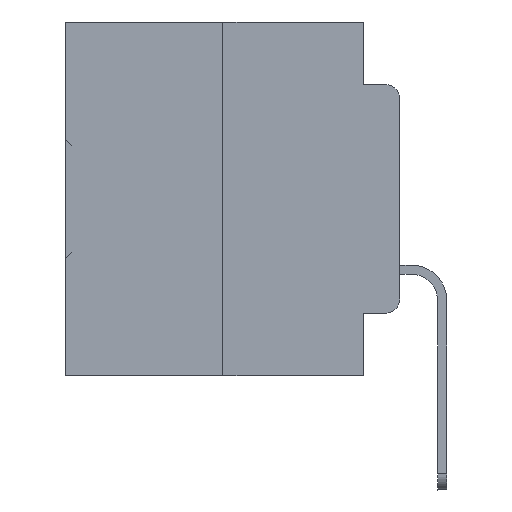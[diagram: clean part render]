
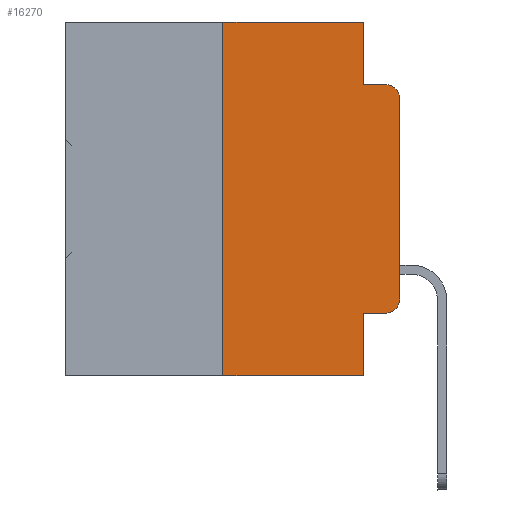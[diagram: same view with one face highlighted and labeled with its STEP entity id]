
A CAD part, left-side view. The second image highlights one B-rep face of the part: STEP entity #16270.
In plain terms, the highlighted planar face has unit normal (-1, 0, 0).
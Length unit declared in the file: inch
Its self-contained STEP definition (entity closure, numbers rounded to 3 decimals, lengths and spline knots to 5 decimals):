
#1047 = DIRECTION ( 'NONE',  ( 0., -1., 0. ) ) ;
#1428 = VERTEX_POINT ( 'NONE', #19701 ) ;
#2067 = AXIS2_PLACEMENT_3D ( 'NONE', #17730, #5120, #20406 ) ;
#2646 = LINE ( 'NONE', #24477, #24398 ) ;
#2714 = VECTOR ( 'NONE', #7329, 39.37008 ) ;
#2801 = CARTESIAN_POINT ( 'NONE',  ( 0., 0.051, -0.4115 ) ) ;
#3658 = CARTESIAN_POINT ( 'NONE',  ( 0., 0.051, 0. ) ) ;
#3923 = EDGE_CURVE ( 'NONE', #4097, #30603, #10318, .T. ) ;
#4097 = VERTEX_POINT ( 'NONE', #33542 ) ;
#4392 = ORIENTED_EDGE ( 'NONE', *, *, #19052, .T. ) ;
#4418 = CARTESIAN_POINT ( 'NONE',  ( 0., 0.473, 0. ) ) ;
#5120 = DIRECTION ( 'NONE',  ( -1., 0., 0. ) ) ;
#6440 = AXIS2_PLACEMENT_3D ( 'NONE', #33816, #31138, #26849 ) ;
#6537 = CARTESIAN_POINT ( 'NONE',  ( 0., 0.051, 0. ) ) ;
#7329 = DIRECTION ( 'NONE',  ( 0., 0., -1. ) ) ;
#7428 = EDGE_CURVE ( 'NONE', #25751, #30376, #25580, .T. ) ;
#8177 = DIRECTION ( 'NONE',  ( 0., 0., -1. ) ) ;
#8266 = CARTESIAN_POINT ( 'NONE',  ( 0., 0., 0. ) ) ;
#8696 = CARTESIAN_POINT ( 'NONE',  ( 0., 0.02, -0.3915 ) ) ;
#10022 = LINE ( 'NONE', #2801, #25629 ) ;
#10318 = LINE ( 'NONE', #4418, #25053 ) ;
#10755 = VECTOR ( 'NONE', #1047, 39.37008 ) ;
#11928 = DIRECTION ( 'NONE',  ( 0., 0., -1. ) ) ;
#12005 = PLANE ( 'NONE',  #6440 ) ;
#12244 = ORIENTED_EDGE ( 'NONE', *, *, #13555, .F. ) ;
#12829 = CIRCLE ( 'NONE', #16283, 0.02 ) ;
#13066 = LINE ( 'NONE', #26654, #2714 ) ;
#13218 = DIRECTION ( 'NONE',  ( 0., 0., 1. ) ) ;
#13371 = DIRECTION ( 'NONE',  ( 0., -1., 0. ) ) ;
#13555 = EDGE_CURVE ( 'NONE', #28451, #1428, #25912, .T. ) ;
#14150 = VERTEX_POINT ( 'NONE', #16201 ) ;
#14521 = CARTESIAN_POINT ( 'NONE',  ( 0., 0.02, -0.4115 ) ) ;
#14811 = ORIENTED_EDGE ( 'NONE', *, *, #21193, .F. ) ;
#16160 = DIRECTION ( 'NONE',  ( 0., 0., 1. ) ) ;
#16201 = CARTESIAN_POINT ( 'NONE',  ( 0., 0., -0.1085 ) ) ;
#16270 = ADVANCED_FACE ( 'NONE', ( #22268 ), #12005, .F. ) ;
#16283 = AXIS2_PLACEMENT_3D ( 'NONE', #8696, #22149, #8177 ) ;
#16570 = VERTEX_POINT ( 'NONE', #20389 ) ;
#16969 = EDGE_CURVE ( 'NONE', #30603, #28451, #33043, .T. ) ;
#17385 = ORIENTED_EDGE ( 'NONE', *, *, #7428, .T. ) ;
#17545 = CARTESIAN_POINT ( 'NONE',  ( 0., 0.473, -0.5 ) ) ;
#17730 = CARTESIAN_POINT ( 'NONE',  ( 0., 0.02, -0.1085 ) ) ;
#18510 = LINE ( 'NONE', #8266, #28901 ) ;
#19052 = EDGE_CURVE ( 'NONE', #24013, #14150, #18510, .T. ) ;
#19184 = VERTEX_POINT ( 'NONE', #14521 ) ;
#19273 = ORIENTED_EDGE ( 'NONE', *, *, #34750, .F. ) ;
#19701 = CARTESIAN_POINT ( 'NONE',  ( 0., 0.02, -0.0885 ) ) ;
#20038 = CARTESIAN_POINT ( 'NONE',  ( 0., 0.051, -0.0885 ) ) ;
#20389 = CARTESIAN_POINT ( 'NONE',  ( 0., 0.051, -0.4115 ) ) ;
#20406 = DIRECTION ( 'NONE',  ( 0., 0., -1. ) ) ;
#21034 = ORIENTED_EDGE ( 'NONE', *, *, #16969, .F. ) ;
#21193 = EDGE_CURVE ( 'NONE', #16570, #30376, #13066, .T. ) ;
#21410 = CARTESIAN_POINT ( 'NONE',  ( 0., 0.051, -0.5 ) ) ;
#22149 = DIRECTION ( 'NONE',  ( -1., 0., 0. ) ) ;
#22268 = FACE_OUTER_BOUND ( 'NONE', #26660, .T. ) ;
#22275 = ORIENTED_EDGE ( 'NONE', *, *, #27135, .T. ) ;
#23628 = VECTOR ( 'NONE', #11928, 39.37008 ) ;
#23956 = EDGE_CURVE ( 'NONE', #16570, #19184, #10022, .T. ) ;
#24013 = VERTEX_POINT ( 'NONE', #27140 ) ;
#24398 = VECTOR ( 'NONE', #13218, 39.37008 ) ;
#24477 = CARTESIAN_POINT ( 'NONE',  ( 0., 0.25, 0. ) ) ;
#25053 = VECTOR ( 'NONE', #29101, 39.37008 ) ;
#25580 = LINE ( 'NONE', #17545, #10755 ) ;
#25629 = VECTOR ( 'NONE', #13371, 39.37008 ) ;
#25751 = VERTEX_POINT ( 'NONE', #32159 ) ;
#25912 = LINE ( 'NONE', #31627, #34396 ) ;
#26654 = CARTESIAN_POINT ( 'NONE',  ( 0., 0.051, 0. ) ) ;
#26660 = EDGE_LOOP ( 'NONE', ( #4392, #27583, #12244, #21034, #34229, #19273, #17385, #14811, #32820, #22275 ) ) ;
#26849 = DIRECTION ( 'NONE',  ( 0., 0., -1. ) ) ;
#27135 = EDGE_CURVE ( 'NONE', #19184, #24013, #12829, .T. ) ;
#27140 = CARTESIAN_POINT ( 'NONE',  ( 0., 0., -0.3915 ) ) ;
#27583 = ORIENTED_EDGE ( 'NONE', *, *, #30368, .T. ) ;
#28451 = VERTEX_POINT ( 'NONE', #20038 ) ;
#28901 = VECTOR ( 'NONE', #16160, 39.37008 ) ;
#29101 = DIRECTION ( 'NONE',  ( 0., -1., 0. ) ) ;
#30368 = EDGE_CURVE ( 'NONE', #14150, #1428, #32911, .T. ) ;
#30376 = VERTEX_POINT ( 'NONE', #21410 ) ;
#30603 = VERTEX_POINT ( 'NONE', #3658 ) ;
#31088 = DIRECTION ( 'NONE',  ( 0., -1., 0. ) ) ;
#31138 = DIRECTION ( 'NONE',  ( 1., 0., 0. ) ) ;
#31627 = CARTESIAN_POINT ( 'NONE',  ( 0., 0.051, -0.0885 ) ) ;
#32159 = CARTESIAN_POINT ( 'NONE',  ( 0., 0.25, -0.5 ) ) ;
#32820 = ORIENTED_EDGE ( 'NONE', *, *, #23956, .T. ) ;
#32911 = CIRCLE ( 'NONE', #2067, 0.02 ) ;
#33043 = LINE ( 'NONE', #6537, #23628 ) ;
#33542 = CARTESIAN_POINT ( 'NONE',  ( 0., 0.25, 0. ) ) ;
#33816 = CARTESIAN_POINT ( 'NONE',  ( 0., 0.473, 0. ) ) ;
#34229 = ORIENTED_EDGE ( 'NONE', *, *, #3923, .F. ) ;
#34396 = VECTOR ( 'NONE', #31088, 39.37008 ) ;
#34750 = EDGE_CURVE ( 'NONE', #25751, #4097, #2646, .T. ) ;
